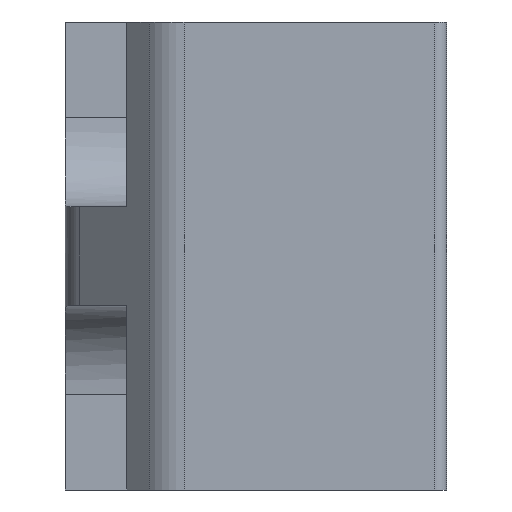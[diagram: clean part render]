
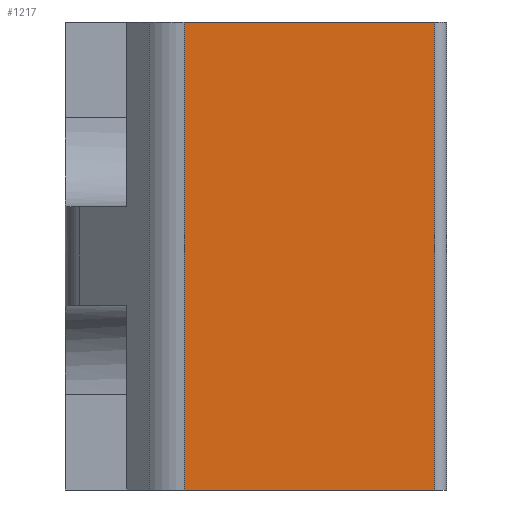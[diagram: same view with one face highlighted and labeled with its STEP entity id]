
A CAD part, front view. The second image highlights one B-rep face of the part: STEP entity #1217.
In plain terms, the highlighted planar face has unit normal (0, -1, 0).
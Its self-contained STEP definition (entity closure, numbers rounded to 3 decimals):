
#124 = ORIENTED_EDGE ( 'NONE', *, *, #882, .T. ) ;
#164 = CARTESIAN_POINT ( 'NONE',  ( -16., -17.5, -19. ) ) ;
#232 = VECTOR ( 'NONE', #1656, 1000. ) ;
#248 = VERTEX_POINT ( 'NONE', #1282 ) ;
#264 = VERTEX_POINT ( 'NONE', #452 ) ;
#322 = CARTESIAN_POINT ( 'NONE',  ( -1., -17.5, -19. ) ) ;
#411 = AXIS2_PLACEMENT_3D ( 'NONE', #164, #856, #1436 ) ;
#440 = LINE ( 'NONE', #1451, #809 ) ;
#452 = CARTESIAN_POINT ( 'NONE',  ( -1., -17.5, 0. ) ) ;
#584 = EDGE_LOOP ( 'NONE', ( #1306, #1286, #1352, #124 ) ) ;
#675 = FACE_OUTER_BOUND ( 'NONE', #584, .T. ) ;
#723 = LINE ( 'NONE', #1576, #1226 ) ;
#767 = DIRECTION ( 'NONE',  ( 0., 0., -1. ) ) ;
#794 = EDGE_CURVE ( 'NONE', #1679, #264, #723, .T. ) ;
#803 = CARTESIAN_POINT ( 'NONE',  ( -11.172, -17.5, 0. ) ) ;
#809 = VECTOR ( 'NONE', #767, 1000. ) ;
#856 = DIRECTION ( 'NONE',  ( 0., -1., 0. ) ) ;
#882 = EDGE_CURVE ( 'NONE', #1679, #248, #440, .T. ) ;
#1059 = EDGE_CURVE ( 'NONE', #248, #1332, #1202, .T. ) ;
#1117 = VECTOR ( 'NONE', #1502, 1000. ) ;
#1202 = LINE ( 'NONE', #1386, #1117 ) ;
#1217 = ADVANCED_FACE ( 'NONE', ( #675 ), #1568, .T. ) ;
#1226 = VECTOR ( 'NONE', #1558, 1000. ) ;
#1228 = LINE ( 'NONE', #1792, #232 ) ;
#1282 = CARTESIAN_POINT ( 'NONE',  ( -11.172, -17.5, -19. ) ) ;
#1286 = ORIENTED_EDGE ( 'NONE', *, *, #1714, .T. ) ;
#1306 = ORIENTED_EDGE ( 'NONE', *, *, #1059, .T. ) ;
#1332 = VERTEX_POINT ( 'NONE', #322 ) ;
#1352 = ORIENTED_EDGE ( 'NONE', *, *, #794, .F. ) ;
#1386 = CARTESIAN_POINT ( 'NONE',  ( -16., -17.5, -19. ) ) ;
#1436 = DIRECTION ( 'NONE',  ( 0., 0., -1. ) ) ;
#1451 = CARTESIAN_POINT ( 'NONE',  ( -11.172, -17.5, -19. ) ) ;
#1502 = DIRECTION ( 'NONE',  ( 1., 0., 0. ) ) ;
#1558 = DIRECTION ( 'NONE',  ( 1., 0., 0. ) ) ;
#1568 = PLANE ( 'NONE',  #411 ) ;
#1576 = CARTESIAN_POINT ( 'NONE',  ( -16., -17.5, 0. ) ) ;
#1656 = DIRECTION ( 'NONE',  ( 0., 0., 1. ) ) ;
#1679 = VERTEX_POINT ( 'NONE', #803 ) ;
#1714 = EDGE_CURVE ( 'NONE', #1332, #264, #1228, .T. ) ;
#1792 = CARTESIAN_POINT ( 'NONE',  ( -1., -17.5, 0. ) ) ;
